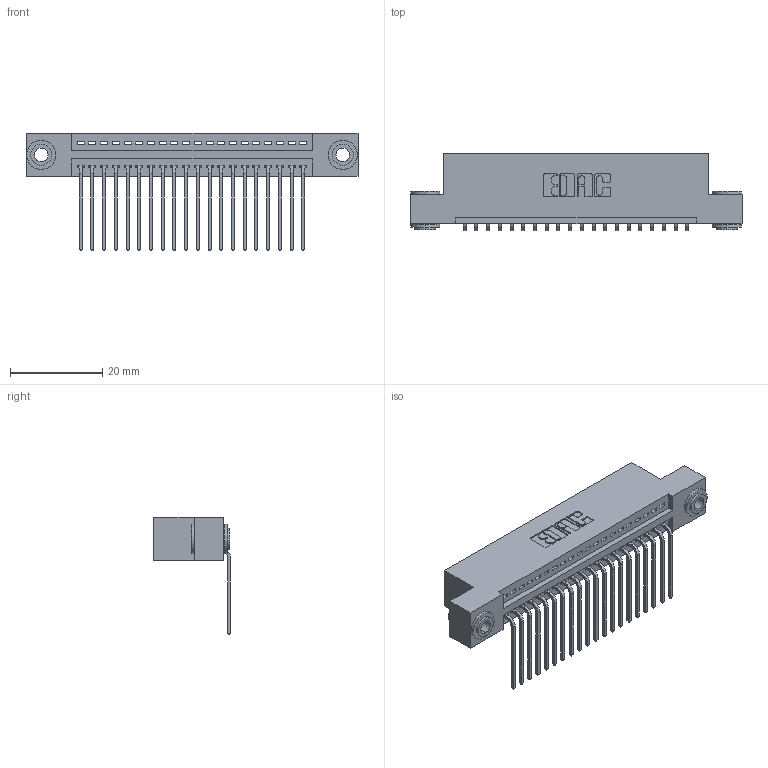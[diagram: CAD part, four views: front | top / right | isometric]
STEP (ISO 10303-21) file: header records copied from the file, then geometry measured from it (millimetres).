
FILE_DESCRIPTION (( 'STEP AP203' ), '1' );
FILE_NAME ('395-020-559-103.STEP', '2019-10-17T19:27:38', ( '' ), ( '' ), 'SwSTEP 2.0', 'SolidWorks 2016', '' );
FILE_SCHEMA (( 'CONFIG_CONTROL_DESIGN' ));
Length unit declared in the file: inch
Products named in the file (4): 395-020-559-103; 345 Part_Flush Mounting Lugs - 0.156 Dia-TH; 345-250-002_345-250-002-102; 345-292-001_558 559 Tail - 1
Assembly tree (23 placements, depth 2):
  395-020-559-103
    345 Part_Flush Mounting Lugs - 0.156 Dia-TH
    345-292-001_558 559 Tail - 1  x20
    345-250-002_345-250-002-102  x2
Bounding box: 72.01 x 16.75 x 25.53 mm (x, y, z)
Volume: 6745.3 mm3; surface area: 9270.9 mm2
Topology: 23 solids, 23 shells, 1364 faces, 4057 edges, 2674 vertices
Faces by surface type: plane 930, cylinder 426, cone 8
Entity records: 18748 total; most frequent: CARTESIAN_POINT 3227, ORIENTED_EDGE 3174, DIRECTION 2881, EDGE_CURVE 1587, VECTOR 1351, LINE 1351, VERTEX_POINT 1054, AXIS2_PLACEMENT_3D 765
